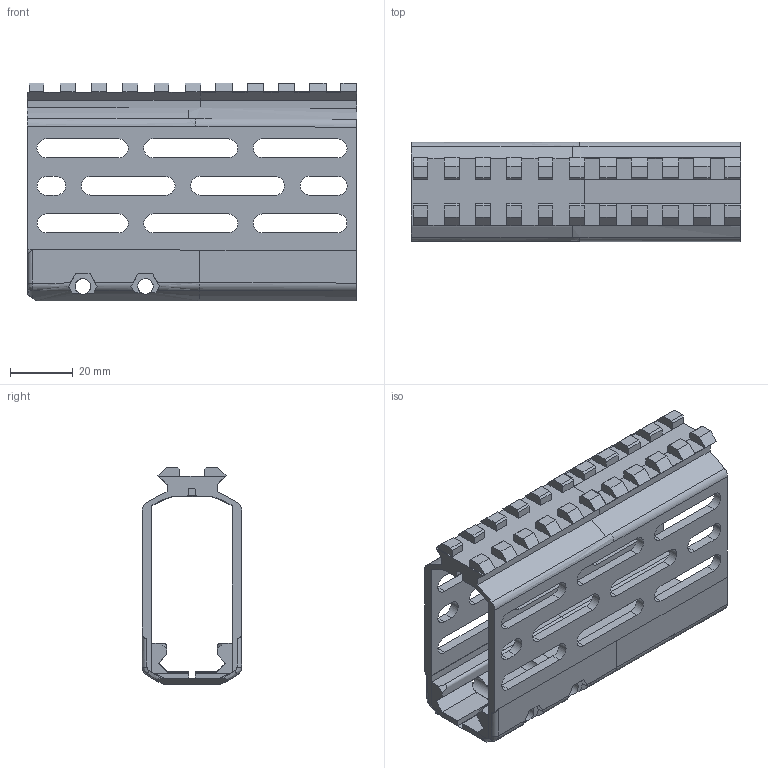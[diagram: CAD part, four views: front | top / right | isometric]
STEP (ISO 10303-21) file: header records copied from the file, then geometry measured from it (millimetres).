
FILE_DESCRIPTION(/* description */ (''),/* implementation_level */ '2;1');
FILE_NAME(/* name */ 'handguard.step',/* time_stamp */ '2021-09-02T19:30:52-05:00',/* author */ (''),/* organization */ (''),/* preprocessor_version */ 'ST-DEVELOPER v18.1',/* originating_system */ 'Autodesk Translation Framework v10.10.0.1391',/* authorisation */ '');
FILE_SCHEMA (('AUTOMOTIVE_DESIGN { 1 0 10303 214 3 1 1 }'));
Length unit declared in the file: millimetre
Products named in the file (1): handguard
Bounding box: 105.27 x 31.81 x 69.71 mm (x, y, z)
Volume: 56917.9 mm3; surface area: 38543.3 mm2
Topology: 1 solids, 1 shells, 394 faces, 1161 edges, 763 vertices
Faces by surface type: plane 286, cylinder 68, bspline 38, torus 2
Full cylindrical faces by diameter (mm): 2.65 x3, 5 x4
Entity records: 14356 total; most frequent: CARTESIAN_POINT 3946, ORIENTED_EDGE 2322, DIRECTION 1920, EDGE_CURVE 1161, LINE 886, VECTOR 886, VERTEX_POINT 763, AXIS2_PLACEMENT_3D 517
